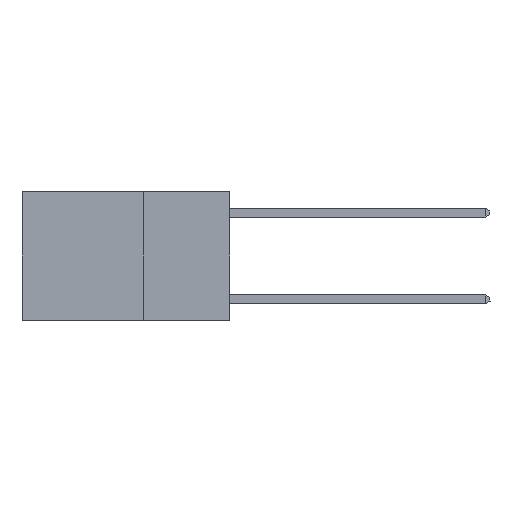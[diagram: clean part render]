
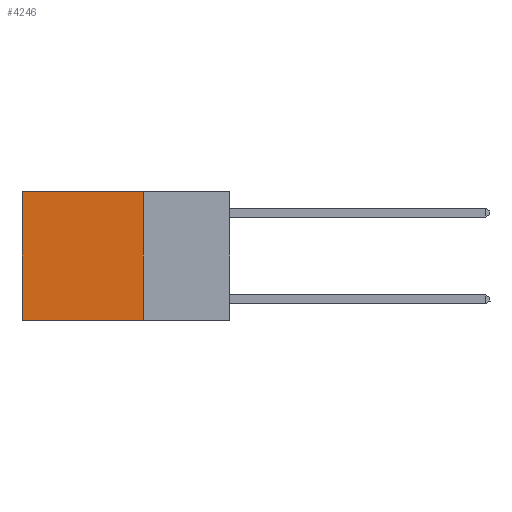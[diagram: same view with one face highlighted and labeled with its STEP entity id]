
A CAD part, left-side view. The second image highlights one B-rep face of the part: STEP entity #4246.
In plain terms, the highlighted planar face has unit normal (-1, 0, 0).
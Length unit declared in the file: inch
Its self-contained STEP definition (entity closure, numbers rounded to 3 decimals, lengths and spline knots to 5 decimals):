
#32 = CARTESIAN_POINT ( 'NONE',  ( 0.2625, 0.25, 0. ) ) ;
#84 = VERTEX_POINT ( 'NONE', #9265 ) ;
#746 = EDGE_CURVE ( 'NONE', #5842, #84, #5268, .T. ) ;
#761 = ORIENTED_EDGE ( 'NONE', *, *, #4145, .F. ) ;
#1565 = ORIENTED_EDGE ( 'NONE', *, *, #5691, .T. ) ;
#2043 = CARTESIAN_POINT ( 'NONE',  ( 0.2625, 0.25, -0.37 ) ) ;
#2047 = AXIS2_PLACEMENT_3D ( 'NONE', #2183, #10439, #4964 ) ;
#2102 = EDGE_LOOP ( 'NONE', ( #1565, #761, #9692, #9702 ) ) ;
#2183 = CARTESIAN_POINT ( 'NONE',  ( 0.2625, 0.25, 0. ) ) ;
#2301 = VERTEX_POINT ( 'NONE', #3285 ) ;
#2513 = EDGE_CURVE ( 'NONE', #5842, #2301, #4549, .T. ) ;
#2793 = VECTOR ( 'NONE', #9609, 39.37008 ) ;
#3285 = CARTESIAN_POINT ( 'NONE',  ( 0.2625, 0.25, -0.37 ) ) ;
#3973 = CARTESIAN_POINT ( 'NONE',  ( 0.2625, 0.6, 0. ) ) ;
#4029 = VECTOR ( 'NONE', #8446, 39.37008 ) ;
#4145 = EDGE_CURVE ( 'NONE', #2301, #8258, #4334, .T. ) ;
#4246 = ADVANCED_FACE ( 'NONE', ( #5351 ), #9545, .F. ) ;
#4334 = LINE ( 'NONE', #2043, #4029 ) ;
#4549 = LINE ( 'NONE', #5903, #6165 ) ;
#4964 = DIRECTION ( 'NONE',  ( 0., 0., -1. ) ) ;
#5268 = LINE ( 'NONE', #32, #2793 ) ;
#5351 = FACE_OUTER_BOUND ( 'NONE', #2102, .T. ) ;
#5691 = EDGE_CURVE ( 'NONE', #84, #8258, #6361, .T. ) ;
#5842 = VERTEX_POINT ( 'NONE', #9807 ) ;
#5903 = CARTESIAN_POINT ( 'NONE',  ( 0.2625, 0.25, 0. ) ) ;
#6165 = VECTOR ( 'NONE', #10209, 39.37008 ) ;
#6361 = LINE ( 'NONE', #3973, #8210 ) ;
#8210 = VECTOR ( 'NONE', #8612, 39.37008 ) ;
#8258 = VERTEX_POINT ( 'NONE', #8432 ) ;
#8432 = CARTESIAN_POINT ( 'NONE',  ( 0.2625, 0.6, -0.37 ) ) ;
#8446 = DIRECTION ( 'NONE',  ( 0., 1., 0. ) ) ;
#8612 = DIRECTION ( 'NONE',  ( 0., 0., -1. ) ) ;
#9265 = CARTESIAN_POINT ( 'NONE',  ( 0.2625, 0.6, 0. ) ) ;
#9545 = PLANE ( 'NONE',  #2047 ) ;
#9609 = DIRECTION ( 'NONE',  ( 0., 1., 0. ) ) ;
#9692 = ORIENTED_EDGE ( 'NONE', *, *, #2513, .F. ) ;
#9702 = ORIENTED_EDGE ( 'NONE', *, *, #746, .T. ) ;
#9807 = CARTESIAN_POINT ( 'NONE',  ( 0.2625, 0.25, 0. ) ) ;
#10209 = DIRECTION ( 'NONE',  ( 0., 0., -1. ) ) ;
#10439 = DIRECTION ( 'NONE',  ( 1., 0., 0. ) ) ;
